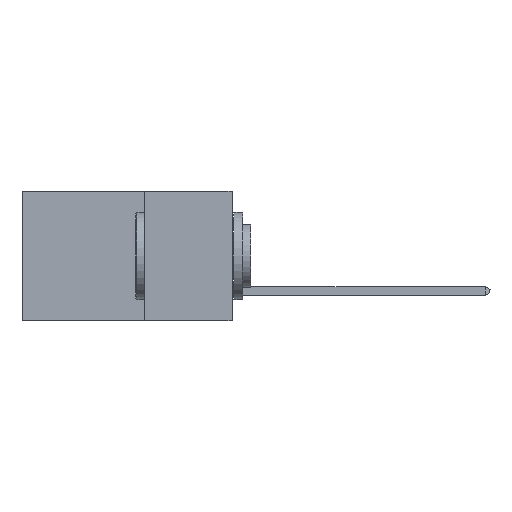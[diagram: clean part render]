
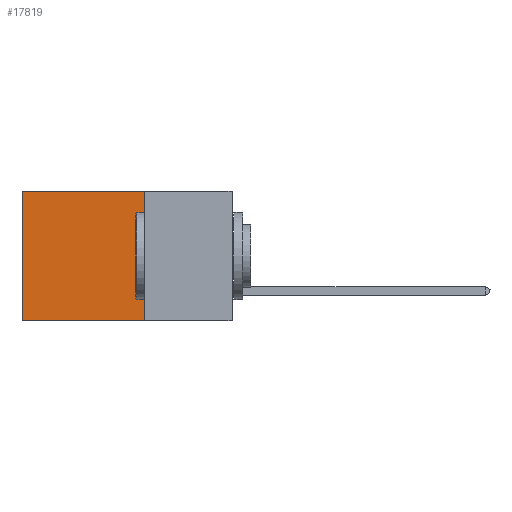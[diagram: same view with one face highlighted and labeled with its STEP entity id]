
A CAD part, left-side view. The second image highlights one B-rep face of the part: STEP entity #17819.
In plain terms, the highlighted planar face has unit normal (-1, 0, 0).
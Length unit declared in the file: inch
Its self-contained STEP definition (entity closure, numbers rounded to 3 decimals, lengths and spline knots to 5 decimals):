
#1397 = CARTESIAN_POINT ( 'NONE',  ( 0.2875, 0.6, 0. ) ) ;
#2022 = CARTESIAN_POINT ( 'NONE',  ( 0.2875, 0.6, -0.37 ) ) ;
#2035 = EDGE_CURVE ( 'NONE', #2567, #2692, #5924, .T. ) ;
#2567 = VERTEX_POINT ( 'NONE', #24261 ) ;
#2692 = VERTEX_POINT ( 'NONE', #8593 ) ;
#2771 = CARTESIAN_POINT ( 'NONE',  ( 0.2875, 0.25, 0. ) ) ;
#4517 = EDGE_CURVE ( 'NONE', #2692, #26606, #6929, .T. ) ;
#5924 = LINE ( 'NONE', #7971, #28495 ) ;
#6929 = LINE ( 'NONE', #20182, #23988 ) ;
#7510 = LINE ( 'NONE', #24509, #15190 ) ;
#7971 = CARTESIAN_POINT ( 'NONE',  ( 0.2875, 0.25, 0. ) ) ;
#8593 = CARTESIAN_POINT ( 'NONE',  ( 0.2875, 0.25, -0.37 ) ) ;
#9364 = EDGE_CURVE ( 'NONE', #11519, #26606, #25191, .T. ) ;
#10545 = DIRECTION ( 'NONE',  ( 0., 1., 0. ) ) ;
#11004 = DIRECTION ( 'NONE',  ( 0., 1., 0. ) ) ;
#11519 = VERTEX_POINT ( 'NONE', #1397 ) ;
#11960 = ORIENTED_EDGE ( 'NONE', *, *, #2035, .F. ) ;
#12151 = DIRECTION ( 'NONE',  ( 1., 0., 0. ) ) ;
#12925 = DIRECTION ( 'NONE',  ( 0., 0., -1. ) ) ;
#13549 = ORIENTED_EDGE ( 'NONE', *, *, #4517, .F. ) ;
#14810 = PLANE ( 'NONE',  #21218 ) ;
#15104 = ORIENTED_EDGE ( 'NONE', *, *, #9364, .T. ) ;
#15190 = VECTOR ( 'NONE', #10545, 39.37008 ) ;
#16585 = ORIENTED_EDGE ( 'NONE', *, *, #26395, .T. ) ;
#16907 = DIRECTION ( 'NONE',  ( 0., 0., -1. ) ) ;
#17357 = CARTESIAN_POINT ( 'NONE',  ( 0.2875, 0.6, 0. ) ) ;
#17819 = ADVANCED_FACE ( 'NONE', ( #23684 ), #14810, .F. ) ;
#20182 = CARTESIAN_POINT ( 'NONE',  ( 0.2875, 0.25, -0.37 ) ) ;
#21218 = AXIS2_PLACEMENT_3D ( 'NONE', #2771, #12151, #26199 ) ;
#21907 = VECTOR ( 'NONE', #12925, 39.37008 ) ;
#22076 = EDGE_LOOP ( 'NONE', ( #15104, #13549, #11960, #16585 ) ) ;
#23684 = FACE_OUTER_BOUND ( 'NONE', #22076, .T. ) ;
#23988 = VECTOR ( 'NONE', #11004, 39.37008 ) ;
#24261 = CARTESIAN_POINT ( 'NONE',  ( 0.2875, 0.25, 0. ) ) ;
#24509 = CARTESIAN_POINT ( 'NONE',  ( 0.2875, 0.25, 0. ) ) ;
#25191 = LINE ( 'NONE', #17357, #21907 ) ;
#26199 = DIRECTION ( 'NONE',  ( 0., 0., -1. ) ) ;
#26395 = EDGE_CURVE ( 'NONE', #2567, #11519, #7510, .T. ) ;
#26606 = VERTEX_POINT ( 'NONE', #2022 ) ;
#28495 = VECTOR ( 'NONE', #16907, 39.37008 ) ;
